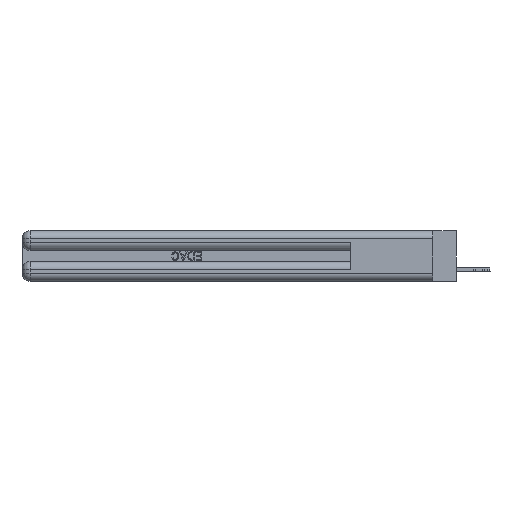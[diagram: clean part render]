
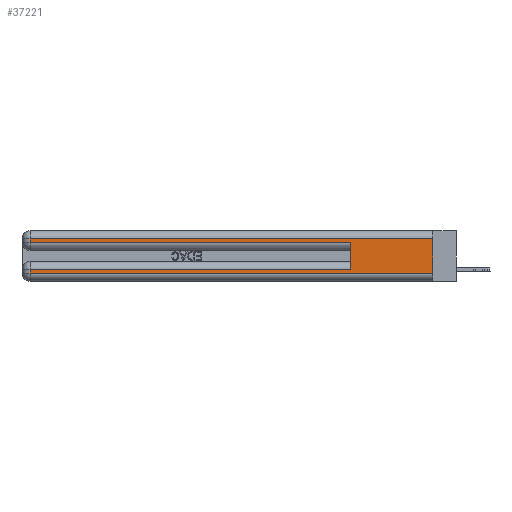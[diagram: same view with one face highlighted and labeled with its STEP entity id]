
A CAD part, left-side view. The second image highlights one B-rep face of the part: STEP entity #37221.
In plain terms, the highlighted planar face has unit normal (-1, 0, 0).
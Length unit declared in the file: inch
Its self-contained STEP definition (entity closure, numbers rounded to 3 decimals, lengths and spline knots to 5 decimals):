
#1630 = LINE ( 'NONE', #7592, #18713 ) ;
#1731 = VECTOR ( 'NONE', #3095, 39.37008 ) ;
#1761 = ORIENTED_EDGE ( 'NONE', *, *, #13397, .T. ) ;
#3095 = DIRECTION ( 'NONE',  ( 0., 1., 0. ) ) ;
#3099 = ORIENTED_EDGE ( 'NONE', *, *, #33727, .T. ) ;
#3159 = CARTESIAN_POINT ( 'NONE',  ( 0., 2.94, 0.37 ) ) ;
#3749 = EDGE_CURVE ( 'NONE', #27760, #15798, #25475, .T. ) ;
#4316 = DIRECTION ( 'NONE',  ( 0., 1., 0. ) ) ;
#4371 = PLANE ( 'NONE',  #9159 ) ;
#4638 = EDGE_LOOP ( 'NONE', ( #17840, #29702, #20960, #3099, #6559, #42357, #1761, #21844 ) ) ;
#4679 = CARTESIAN_POINT ( 'NONE',  ( 0., 2.94, 0.06 ) ) ;
#4684 = DIRECTION ( 'NONE',  ( 0., 0., -1. ) ) ;
#6277 = LINE ( 'NONE', #16126, #11153 ) ;
#6559 = ORIENTED_EDGE ( 'NONE', *, *, #20570, .F. ) ;
#7592 = CARTESIAN_POINT ( 'NONE',  ( 0., 0., 0.085 ) ) ;
#9159 = AXIS2_PLACEMENT_3D ( 'NONE', #32622, #43294, #4684 ) ;
#9917 = VECTOR ( 'NONE', #19245, 39.37008 ) ;
#11001 = EDGE_CURVE ( 'NONE', #27760, #42918, #45259, .T. ) ;
#11153 = VECTOR ( 'NONE', #19685, 39.37008 ) ;
#12303 = EDGE_CURVE ( 'NONE', #31006, #39256, #1630, .T. ) ;
#13397 = EDGE_CURVE ( 'NONE', #39256, #24129, #41197, .T. ) ;
#15424 = FACE_OUTER_BOUND ( 'NONE', #4638, .T. ) ;
#15798 = VERTEX_POINT ( 'NONE', #33002 ) ;
#16126 = CARTESIAN_POINT ( 'NONE',  ( 0., 0., 0.06 ) ) ;
#16137 = VECTOR ( 'NONE', #33187, 39.37008 ) ;
#17840 = ORIENTED_EDGE ( 'NONE', *, *, #11001, .F. ) ;
#18047 = VERTEX_POINT ( 'NONE', #45318 ) ;
#18713 = VECTOR ( 'NONE', #4316, 39.37008 ) ;
#19245 = DIRECTION ( 'NONE',  ( 0., 0., 1. ) ) ;
#19685 = DIRECTION ( 'NONE',  ( 0., -1., 0. ) ) ;
#20570 = EDGE_CURVE ( 'NONE', #31006, #32215, #30965, .T. ) ;
#20960 = ORIENTED_EDGE ( 'NONE', *, *, #27751, .T. ) ;
#21844 = ORIENTED_EDGE ( 'NONE', *, *, #35636, .T. ) ;
#22606 = DIRECTION ( 'NONE',  ( 0., -1., 0. ) ) ;
#24078 = CARTESIAN_POINT ( 'NONE',  ( 0., 0., 0.31 ) ) ;
#24129 = VERTEX_POINT ( 'NONE', #4679 ) ;
#24666 = VECTOR ( 'NONE', #22606, 39.37008 ) ;
#25073 = VECTOR ( 'NONE', #44965, 39.37008 ) ;
#25475 = LINE ( 'NONE', #24078, #1731 ) ;
#26958 = CARTESIAN_POINT ( 'NONE',  ( 0., 0., 0.31 ) ) ;
#27751 = EDGE_CURVE ( 'NONE', #15798, #18047, #38808, .T. ) ;
#27760 = VERTEX_POINT ( 'NONE', #26958 ) ;
#29702 = ORIENTED_EDGE ( 'NONE', *, *, #3749, .T. ) ;
#29794 = CARTESIAN_POINT ( 'NONE',  ( 0., 0.6, 0.085 ) ) ;
#29915 = CARTESIAN_POINT ( 'NONE',  ( 0., 2.94, 0.085 ) ) ;
#30635 = CARTESIAN_POINT ( 'NONE',  ( 0., 0.6, 0.285 ) ) ;
#30965 = LINE ( 'NONE', #35878, #9917 ) ;
#31006 = VERTEX_POINT ( 'NONE', #29794 ) ;
#31099 = CARTESIAN_POINT ( 'NONE',  ( 0., 2.94, 0.37 ) ) ;
#32215 = VERTEX_POINT ( 'NONE', #30635 ) ;
#32622 = CARTESIAN_POINT ( 'NONE',  ( 0., 0., 0.37 ) ) ;
#33002 = CARTESIAN_POINT ( 'NONE',  ( 0., 2.94, 0.31 ) ) ;
#33033 = CARTESIAN_POINT ( 'NONE',  ( 0., 0., 0.37 ) ) ;
#33187 = DIRECTION ( 'NONE',  ( 0., 0., -1. ) ) ;
#33727 = EDGE_CURVE ( 'NONE', #18047, #32215, #33992, .T. ) ;
#33992 = LINE ( 'NONE', #36153, #24666 ) ;
#34602 = DIRECTION ( 'NONE',  ( 0., 0., -1. ) ) ;
#35636 = EDGE_CURVE ( 'NONE', #24129, #42918, #6277, .T. ) ;
#35878 = CARTESIAN_POINT ( 'NONE',  ( 0., 0.6, 0.145 ) ) ;
#36153 = CARTESIAN_POINT ( 'NONE',  ( 0., 0., 0.285 ) ) ;
#37221 = ADVANCED_FACE ( 'NONE', ( #15424 ), #4371, .F. ) ;
#38808 = LINE ( 'NONE', #31099, #25073 ) ;
#39256 = VERTEX_POINT ( 'NONE', #29915 ) ;
#41197 = LINE ( 'NONE', #3159, #42801 ) ;
#41680 = CARTESIAN_POINT ( 'NONE',  ( 0., 0., 0.06 ) ) ;
#42357 = ORIENTED_EDGE ( 'NONE', *, *, #12303, .T. ) ;
#42801 = VECTOR ( 'NONE', #34602, 39.37008 ) ;
#42918 = VERTEX_POINT ( 'NONE', #41680 ) ;
#43294 = DIRECTION ( 'NONE',  ( 1., 0., 0. ) ) ;
#44965 = DIRECTION ( 'NONE',  ( 0., 0., -1. ) ) ;
#45259 = LINE ( 'NONE', #33033, #16137 ) ;
#45318 = CARTESIAN_POINT ( 'NONE',  ( 0., 2.94, 0.285 ) ) ;
